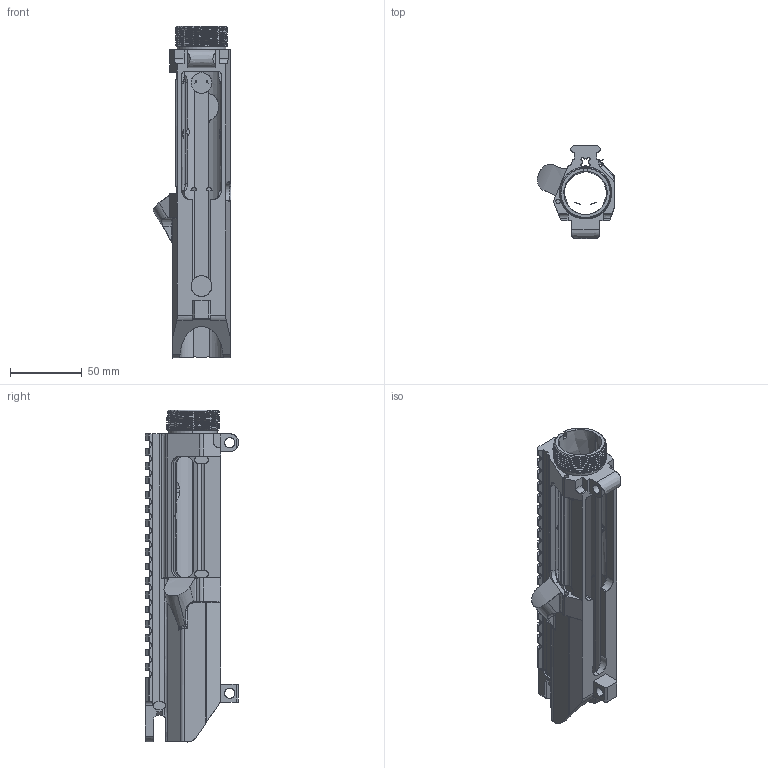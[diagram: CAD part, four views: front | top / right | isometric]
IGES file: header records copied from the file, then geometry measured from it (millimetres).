
Start section: SolidWorks IGES file using analytic representation for surfaces
Global section: file name: WX UPPER.IGS; native system: SolidWorks 2015; preprocessor: SolidWorks 2015; author: WarFairy; date: 160423.092331; units: inch
Bounding box: 53.91 x 65.07 x 231.52 mm (x, y, z)
Surface area: 66854.7 mm2 (no closed solid volume)
Topology: 0 solids, 0 shells, 502 faces, 6240 edges, 6234 vertices
Faces by surface type: bspline 321, revolution 181
